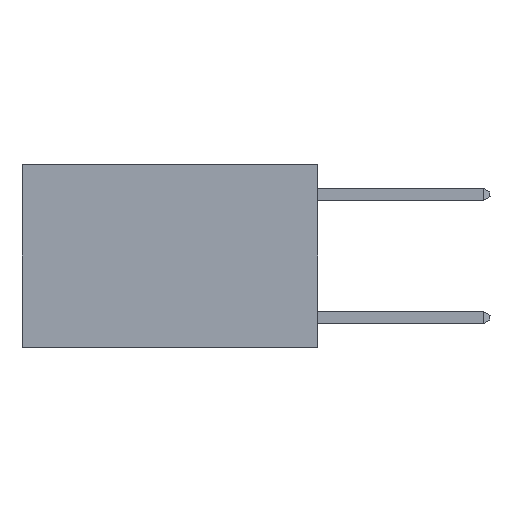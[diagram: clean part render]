
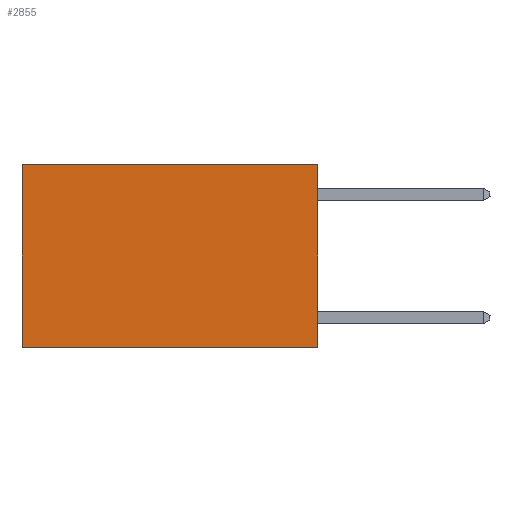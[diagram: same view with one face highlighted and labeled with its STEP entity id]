
A CAD part, left-side view. The second image highlights one B-rep face of the part: STEP entity #2855.
In plain terms, the highlighted planar face has unit normal (-1, 0, 0).
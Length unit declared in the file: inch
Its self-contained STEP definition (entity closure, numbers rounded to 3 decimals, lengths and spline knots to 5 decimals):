
#234 = EDGE_CURVE ( 'NONE', #6992, #1820, #15348, .T. ) ;
#304 = EDGE_CURVE ( 'NONE', #1820, #10373, #5585, .T. ) ;
#437 = DIRECTION ( 'NONE',  ( 1., 0., 0. ) ) ;
#549 = DIRECTION ( 'NONE',  ( 0., 0., -1. ) ) ;
#1310 = VECTOR ( 'NONE', #18340, 39.37008 ) ;
#1820 = VERTEX_POINT ( 'NONE', #16392 ) ;
#2262 = VECTOR ( 'NONE', #18386, 39.37008 ) ;
#2799 = CARTESIAN_POINT ( 'NONE',  ( 0.2625, 0., -0.37 ) ) ;
#2855 = ADVANCED_FACE ( 'NONE', ( #6112 ), #18734, .F. ) ;
#3025 = ORIENTED_EDGE ( 'NONE', *, *, #12866, .F. ) ;
#4523 = DIRECTION ( 'NONE',  ( 0., 0., -1. ) ) ;
#5585 = LINE ( 'NONE', #12827, #19324 ) ;
#5780 = ORIENTED_EDGE ( 'NONE', *, *, #234, .T. ) ;
#6112 = FACE_OUTER_BOUND ( 'NONE', #13244, .T. ) ;
#6262 = CARTESIAN_POINT ( 'NONE',  ( 0.2625, 0., 0. ) ) ;
#6992 = VERTEX_POINT ( 'NONE', #16096 ) ;
#7696 = ORIENTED_EDGE ( 'NONE', *, *, #13804, .F. ) ;
#8524 = CARTESIAN_POINT ( 'NONE',  ( 0.2625, 0., 0. ) ) ;
#8765 = VECTOR ( 'NONE', #17346, 39.37008 ) ;
#8773 = CARTESIAN_POINT ( 'NONE',  ( 0.2625, 0.6, -0.37 ) ) ;
#10373 = VERTEX_POINT ( 'NONE', #8773 ) ;
#11324 = AXIS2_PLACEMENT_3D ( 'NONE', #8524, #437, #549 ) ;
#12044 = VERTEX_POINT ( 'NONE', #15739 ) ;
#12827 = CARTESIAN_POINT ( 'NONE',  ( 0.2625, 0.6, 0. ) ) ;
#12866 = EDGE_CURVE ( 'NONE', #6992, #12044, #18678, .T. ) ;
#13244 = EDGE_LOOP ( 'NONE', ( #19504, #7696, #3025, #5780 ) ) ;
#13804 = EDGE_CURVE ( 'NONE', #12044, #10373, #19800, .T. ) ;
#15348 = LINE ( 'NONE', #6262, #8765 ) ;
#15739 = CARTESIAN_POINT ( 'NONE',  ( 0.2625, 0., -0.37 ) ) ;
#16096 = CARTESIAN_POINT ( 'NONE',  ( 0.2625, 0., 0. ) ) ;
#16392 = CARTESIAN_POINT ( 'NONE',  ( 0.2625, 0.6, 0. ) ) ;
#17346 = DIRECTION ( 'NONE',  ( 0., 1., 0. ) ) ;
#18287 = CARTESIAN_POINT ( 'NONE',  ( 0.2625, 0., 0. ) ) ;
#18340 = DIRECTION ( 'NONE',  ( 0., 1., 0. ) ) ;
#18386 = DIRECTION ( 'NONE',  ( 0., 0., -1. ) ) ;
#18678 = LINE ( 'NONE', #18287, #2262 ) ;
#18734 = PLANE ( 'NONE',  #11324 ) ;
#19324 = VECTOR ( 'NONE', #4523, 39.37008 ) ;
#19504 = ORIENTED_EDGE ( 'NONE', *, *, #304, .T. ) ;
#19800 = LINE ( 'NONE', #2799, #1310 ) ;
